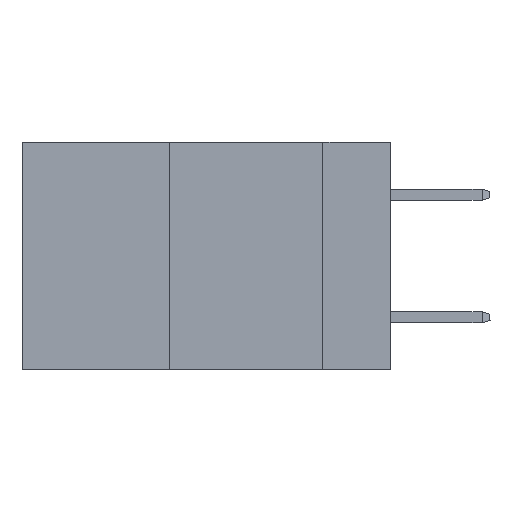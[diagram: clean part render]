
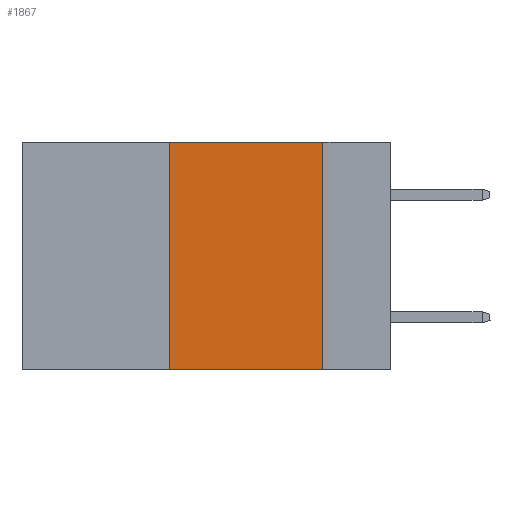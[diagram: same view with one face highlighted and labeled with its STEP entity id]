
A CAD part, left-side view. The second image highlights one B-rep face of the part: STEP entity #1867.
In plain terms, the highlighted planar face has unit normal (-1, 0, 0).
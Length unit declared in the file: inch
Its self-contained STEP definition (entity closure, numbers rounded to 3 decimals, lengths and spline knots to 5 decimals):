
#348 = CARTESIAN_POINT ( 'NONE',  ( 0., 0.11, 0. ) ) ;
#990 = CARTESIAN_POINT ( 'NONE',  ( 0., 0.6, 0. ) ) ;
#1644 = DIRECTION ( 'NONE',  ( 0., 0., 1. ) ) ;
#1795 = VERTEX_POINT ( 'NONE', #25813 ) ;
#1867 = ADVANCED_FACE ( 'NONE', ( #24794 ), #13724, .F. ) ;
#1908 = DIRECTION ( 'NONE',  ( 1., 0., 0. ) ) ;
#4140 = VERTEX_POINT ( 'NONE', #23086 ) ;
#4281 = LINE ( 'NONE', #990, #22434 ) ;
#4873 = VERTEX_POINT ( 'NONE', #25415 ) ;
#7845 = CARTESIAN_POINT ( 'NONE',  ( 0., 0.6, 0. ) ) ;
#7953 = EDGE_CURVE ( 'NONE', #4140, #1795, #21381, .T. ) ;
#8478 = ORIENTED_EDGE ( 'NONE', *, *, #7953, .F. ) ;
#12416 = EDGE_CURVE ( 'NONE', #4140, #4873, #13792, .T. ) ;
#12505 = VECTOR ( 'NONE', #23430, 39.37008 ) ;
#12713 = DIRECTION ( 'NONE',  ( 0., -1., 0. ) ) ;
#13724 = PLANE ( 'NONE',  #17522 ) ;
#13792 = LINE ( 'NONE', #23522, #12505 ) ;
#15045 = VERTEX_POINT ( 'NONE', #348 ) ;
#16477 = EDGE_CURVE ( 'NONE', #15045, #4873, #25762, .T. ) ;
#17522 = AXIS2_PLACEMENT_3D ( 'NONE', #7845, #1908, #19884 ) ;
#18227 = CARTESIAN_POINT ( 'NONE',  ( 0., 0.11, 0. ) ) ;
#19880 = CARTESIAN_POINT ( 'NONE',  ( 0., 0.36, 0. ) ) ;
#19884 = DIRECTION ( 'NONE',  ( 0., 0., -1. ) ) ;
#20080 = VECTOR ( 'NONE', #23531, 39.37008 ) ;
#20736 = VECTOR ( 'NONE', #1644, 39.37008 ) ;
#21381 = LINE ( 'NONE', #19880, #20736 ) ;
#22031 = ORIENTED_EDGE ( 'NONE', *, *, #23754, .F. ) ;
#22434 = VECTOR ( 'NONE', #12713, 39.37008 ) ;
#23086 = CARTESIAN_POINT ( 'NONE',  ( 0., 0.36, -0.37 ) ) ;
#23430 = DIRECTION ( 'NONE',  ( 0., -1., 0. ) ) ;
#23522 = CARTESIAN_POINT ( 'NONE',  ( 0., 0.6, -0.37 ) ) ;
#23531 = DIRECTION ( 'NONE',  ( 0., 0., -1. ) ) ;
#23754 = EDGE_CURVE ( 'NONE', #1795, #15045, #4281, .T. ) ;
#24007 = ORIENTED_EDGE ( 'NONE', *, *, #16477, .F. ) ;
#24310 = EDGE_LOOP ( 'NONE', ( #24007, #22031, #8478, #25364 ) ) ;
#24794 = FACE_OUTER_BOUND ( 'NONE', #24310, .T. ) ;
#25364 = ORIENTED_EDGE ( 'NONE', *, *, #12416, .T. ) ;
#25415 = CARTESIAN_POINT ( 'NONE',  ( 0., 0.11, -0.37 ) ) ;
#25762 = LINE ( 'NONE', #18227, #20080 ) ;
#25813 = CARTESIAN_POINT ( 'NONE',  ( 0., 0.36, 0. ) ) ;
